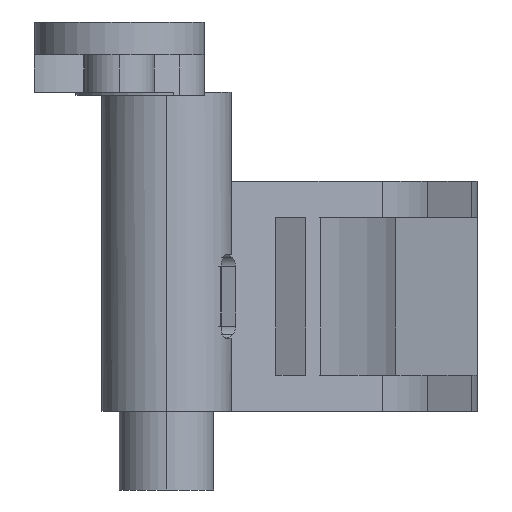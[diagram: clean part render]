
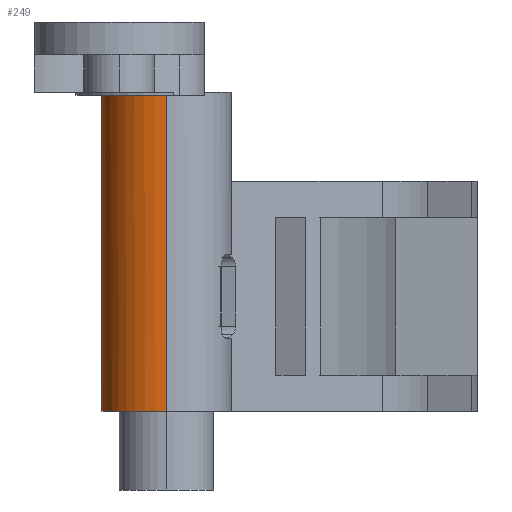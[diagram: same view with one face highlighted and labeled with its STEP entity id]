
A CAD part, left-side view. The second image highlights one B-rep face of the part: STEP entity #249.
In plain terms, the highlighted cylindrical face has radius 2.686 mm (diameter 5.372 mm), a partial arc.
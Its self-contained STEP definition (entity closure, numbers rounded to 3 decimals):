
#208 = ORIENTED_EDGE ( 'NONE', *, *, #287, .T. ) ;
#235 = EDGE_CURVE ( 'NONE', #2512, #1964, #2658, .T. ) ;
#242 = CARTESIAN_POINT ( 'NONE',  ( 11.746, -1.454, 8.319 ) ) ;
#249 = ADVANCED_FACE ( 'NONE', ( #524 ), #1639, .T. ) ;
#255 = EDGE_CURVE ( 'NONE', #1964, #375, #2617, .T. ) ;
#263 = CARTESIAN_POINT ( 'NONE',  ( 6.419, -1.943, -4.762 ) ) ;
#275 = EDGE_CURVE ( 'NONE', #375, #1847, #2172, .T. ) ;
#287 = EDGE_CURVE ( 'NONE', #1847, #1414, #2566, .T. ) ;
#315 = EDGE_CURVE ( 'NONE', #1042, #1414, #2524, .T. ) ;
#357 = ORIENTED_EDGE ( 'NONE', *, *, #315, .F. ) ;
#359 = EDGE_CURVE ( 'NONE', #782, #1042, #1989, .T. ) ;
#372 = EDGE_CURVE ( 'NONE', #1285, #782, #2471, .T. ) ;
#375 = VERTEX_POINT ( 'NONE', #800 ) ;
#391 = EDGE_CURVE ( 'NONE', #1285, #2512, #922, .T. ) ;
#524 = FACE_OUTER_BOUND ( 'NONE', #2125, .T. ) ;
#601 = ORIENTED_EDGE ( 'NONE', *, *, #255, .T. ) ;
#653 = CARTESIAN_POINT ( 'NONE',  ( 9.105, -1.943, 4.762 ) ) ;
#660 = DIRECTION ( 'NONE',  ( 0., 0., -1. ) ) ;
#671 = CARTESIAN_POINT ( 'NONE',  ( 11.495, -0.717, 0. ) ) ;
#696 = CARTESIAN_POINT ( 'NONE',  ( 11.746, -1.454, 11.354 ) ) ;
#699 = DIRECTION ( 'NONE',  ( 0.544, -0.839, 0. ) ) ;
#703 = DIRECTION ( 'NONE',  ( 0., 0., -1. ) ) ;
#724 = DIRECTION ( 'NONE',  ( 0., 0., 1. ) ) ;
#768 = CARTESIAN_POINT ( 'NONE',  ( 11.791, -1.943, -4.762 ) ) ;
#782 = VERTEX_POINT ( 'NONE', #1770 ) ;
#792 = CARTESIAN_POINT ( 'NONE',  ( 11.495, -0.717, -4.762 ) ) ;
#800 = CARTESIAN_POINT ( 'NONE',  ( 6.419, -1.943, 8.319 ) ) ;
#922 = LINE ( 'NONE', #671, #2405 ) ;
#947 = CARTESIAN_POINT ( 'NONE',  ( 11.495, -0.717, 4.762 ) ) ;
#1027 = ORIENTED_EDGE ( 'NONE', *, *, #359, .F. ) ;
#1042 = VERTEX_POINT ( 'NONE', #1333 ) ;
#1060 = DIRECTION ( 'NONE',  ( 0.81, -0.586, 0. ) ) ;
#1063 = DIRECTION ( 'NONE',  ( 0., 0., 1. ) ) ;
#1085 = CARTESIAN_POINT ( 'NONE',  ( 9.105, -1.943, 11.354 ) ) ;
#1124 = VECTOR ( 'NONE', #1569, 1000. ) ;
#1156 = ORIENTED_EDGE ( 'NONE', *, *, #391, .T. ) ;
#1196 = DIRECTION ( 'NONE',  ( 0., 0., 1. ) ) ;
#1262 = CARTESIAN_POINT ( 'NONE',  ( 9.105, -1.943, 8.319 ) ) ;
#1266 = DIRECTION ( 'NONE',  ( 1., 0., 0. ) ) ;
#1269 = DIRECTION ( 'NONE',  ( 0., 0., -1. ) ) ;
#1285 = VERTEX_POINT ( 'NONE', #947 ) ;
#1333 = CARTESIAN_POINT ( 'NONE',  ( 11.791, -1.943, 11.354 ) ) ;
#1414 = VERTEX_POINT ( 'NONE', #696 ) ;
#1425 = VECTOR ( 'NONE', #724, 1000. ) ;
#1533 = CARTESIAN_POINT ( 'NONE',  ( 9.105, -1.943, -4.762 ) ) ;
#1552 = CARTESIAN_POINT ( 'NONE',  ( 11.746, -1.454, -4.762 ) ) ;
#1558 = DIRECTION ( 'NONE',  ( 1., 0., 0. ) ) ;
#1566 = CARTESIAN_POINT ( 'NONE',  ( 6.419, -1.943, -4.762 ) ) ;
#1569 = DIRECTION ( 'NONE',  ( 0., 0., 1. ) ) ;
#1572 = DIRECTION ( 'NONE',  ( 0., 0., 1. ) ) ;
#1579 = DIRECTION ( 'NONE',  ( 1., 0., 0. ) ) ;
#1588 = DIRECTION ( 'NONE',  ( 0., 0., 1. ) ) ;
#1600 = CARTESIAN_POINT ( 'NONE',  ( 9.105, -1.943, -4.762 ) ) ;
#1639 = CYLINDRICAL_SURFACE ( 'NONE', #2014, 2.686 ) ;
#1644 = ORIENTED_EDGE ( 'NONE', *, *, #235, .T. ) ;
#1770 = CARTESIAN_POINT ( 'NONE',  ( 11.791, -1.943, 4.762 ) ) ;
#1847 = VERTEX_POINT ( 'NONE', #242 ) ;
#1929 = AXIS2_PLACEMENT_3D ( 'NONE', #653, #703, #699 ) ;
#1948 = AXIS2_PLACEMENT_3D ( 'NONE', #1085, #1063, #1060 ) ;
#1964 = VERTEX_POINT ( 'NONE', #263 ) ;
#1989 = LINE ( 'NONE', #768, #1425 ) ;
#2014 = AXIS2_PLACEMENT_3D ( 'NONE', #1533, #1588, #1579 ) ;
#2019 = AXIS2_PLACEMENT_3D ( 'NONE', #1262, #1269, #1266 ) ;
#2053 = VECTOR ( 'NONE', #1196, 1000. ) ;
#2067 = AXIS2_PLACEMENT_3D ( 'NONE', #1600, #1572, #1558 ) ;
#2125 = EDGE_LOOP ( 'NONE', ( #1644, #601, #2323, #208, #357, #1027, #2599, #1156 ) ) ;
#2172 = CIRCLE ( 'NONE', #2019, 2.686 ) ;
#2323 = ORIENTED_EDGE ( 'NONE', *, *, #275, .T. ) ;
#2405 = VECTOR ( 'NONE', #660, 1000. ) ;
#2471 = CIRCLE ( 'NONE', #1929, 2.686 ) ;
#2512 = VERTEX_POINT ( 'NONE', #792 ) ;
#2524 = CIRCLE ( 'NONE', #1948, 2.686 ) ;
#2566 = LINE ( 'NONE', #1552, #2053 ) ;
#2599 = ORIENTED_EDGE ( 'NONE', *, *, #372, .F. ) ;
#2617 = LINE ( 'NONE', #1566, #1124 ) ;
#2658 = CIRCLE ( 'NONE', #2067, 2.686 ) ;
